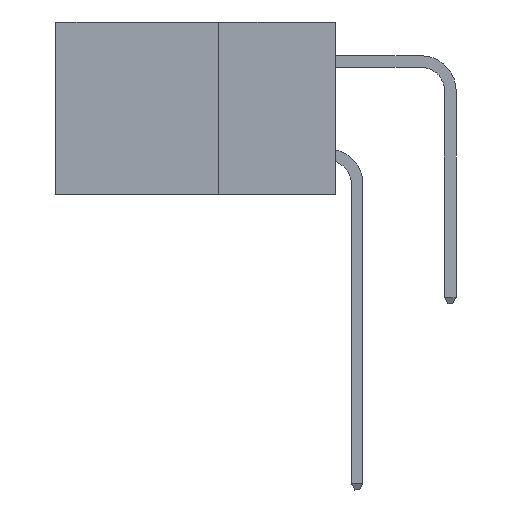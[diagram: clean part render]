
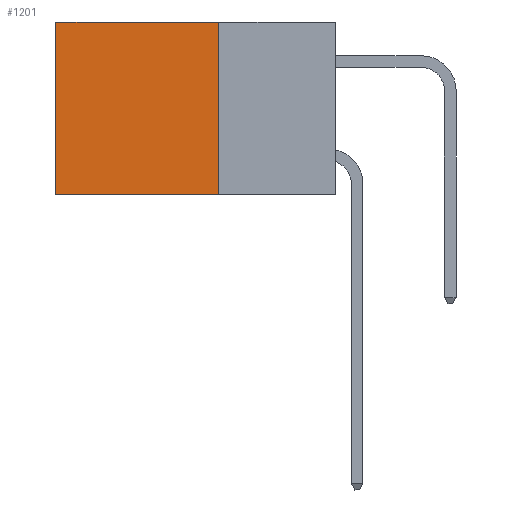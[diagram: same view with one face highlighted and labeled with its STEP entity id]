
A CAD part, left-side view. The second image highlights one B-rep face of the part: STEP entity #1201.
In plain terms, the highlighted planar face has unit normal (-1, 0, 0).
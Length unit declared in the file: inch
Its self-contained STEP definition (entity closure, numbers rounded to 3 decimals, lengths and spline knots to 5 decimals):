
#1201 = ADVANCED_FACE ( 'NONE', ( #28382 ), #24448, .F. ) ;
#1505 = DIRECTION ( 'NONE',  ( 0., 1., 0. ) ) ;
#1546 = EDGE_CURVE ( 'NONE', #36509, #11014, #29848, .T. ) ;
#1571 = DIRECTION ( 'NONE',  ( 1., 0., 0. ) ) ;
#2019 = EDGE_CURVE ( 'NONE', #11014, #28112, #5177, .T. ) ;
#2496 = VECTOR ( 'NONE', #1505, 39.37008 ) ;
#4262 = VECTOR ( 'NONE', #10580, 39.37008 ) ;
#4371 = EDGE_CURVE ( 'NONE', #19300, #28112, #41232, .T. ) ;
#4531 = CARTESIAN_POINT ( 'NONE',  ( 0.2875, 0.25, 0. ) ) ;
#5177 = LINE ( 'NONE', #25937, #23305 ) ;
#5793 = ORIENTED_EDGE ( 'NONE', *, *, #22634, .F. ) ;
#8959 = DIRECTION ( 'NONE',  ( 0., 0., -1. ) ) ;
#10115 = CARTESIAN_POINT ( 'NONE',  ( 0.2875, 0.25, -0.37 ) ) ;
#10580 = DIRECTION ( 'NONE',  ( 0., 1., 0. ) ) ;
#11014 = VERTEX_POINT ( 'NONE', #21215 ) ;
#14274 = EDGE_LOOP ( 'NONE', ( #15509, #21365, #5793, #40321 ) ) ;
#15509 = ORIENTED_EDGE ( 'NONE', *, *, #2019, .T. ) ;
#17527 = CARTESIAN_POINT ( 'NONE',  ( 0.2875, 0.25, -0.37 ) ) ;
#17800 = LINE ( 'NONE', #39673, #34869 ) ;
#19300 = VERTEX_POINT ( 'NONE', #10115 ) ;
#21215 = CARTESIAN_POINT ( 'NONE',  ( 0.2875, 0.6, 0. ) ) ;
#21365 = ORIENTED_EDGE ( 'NONE', *, *, #4371, .F. ) ;
#22634 = EDGE_CURVE ( 'NONE', #36509, #19300, #17800, .T. ) ;
#23305 = VECTOR ( 'NONE', #8959, 39.37008 ) ;
#23534 = DIRECTION ( 'NONE',  ( 0., 0., -1. ) ) ;
#23921 = DIRECTION ( 'NONE',  ( 0., 0., -1. ) ) ;
#24448 = PLANE ( 'NONE',  #38643 ) ;
#25937 = CARTESIAN_POINT ( 'NONE',  ( 0.2875, 0.6, 0. ) ) ;
#28112 = VERTEX_POINT ( 'NONE', #39593 ) ;
#28382 = FACE_OUTER_BOUND ( 'NONE', #14274, .T. ) ;
#29848 = LINE ( 'NONE', #4531, #4262 ) ;
#31378 = CARTESIAN_POINT ( 'NONE',  ( 0.2875, 0.25, 0. ) ) ;
#33433 = CARTESIAN_POINT ( 'NONE',  ( 0.2875, 0.25, 0. ) ) ;
#34869 = VECTOR ( 'NONE', #23534, 39.37008 ) ;
#36509 = VERTEX_POINT ( 'NONE', #31378 ) ;
#38643 = AXIS2_PLACEMENT_3D ( 'NONE', #33433, #1571, #23921 ) ;
#39593 = CARTESIAN_POINT ( 'NONE',  ( 0.2875, 0.6, -0.37 ) ) ;
#39673 = CARTESIAN_POINT ( 'NONE',  ( 0.2875, 0.25, 0. ) ) ;
#40321 = ORIENTED_EDGE ( 'NONE', *, *, #1546, .T. ) ;
#41232 = LINE ( 'NONE', #17527, #2496 ) ;
